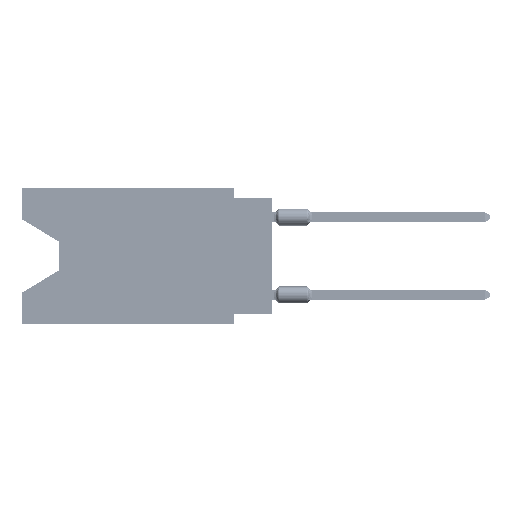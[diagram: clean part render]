
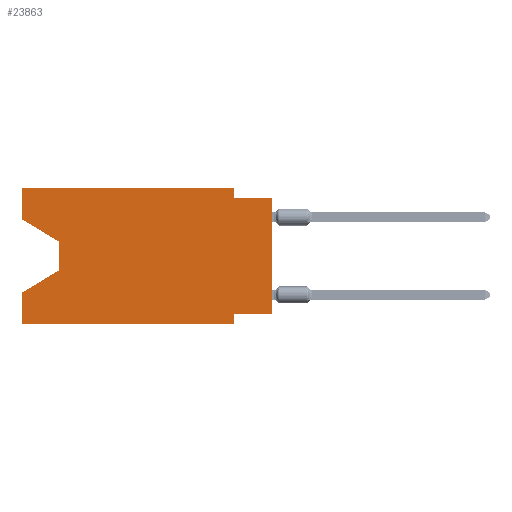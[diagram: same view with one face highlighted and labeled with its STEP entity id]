
A CAD part, left-side view. The second image highlights one B-rep face of the part: STEP entity #23863.
In plain terms, the highlighted planar face has unit normal (-1, 0, 0).
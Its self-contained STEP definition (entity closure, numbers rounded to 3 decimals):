
#1742 = CARTESIAN_POINT ( 'NONE',  ( 0., 2.54, -8.255 ) ) ;
#2446 = VECTOR ( 'NONE', #30770, 1000. ) ;
#2973 = CARTESIAN_POINT ( 'NONE',  ( 0., 16.383, -8.89 ) ) ;
#3612 = LINE ( 'NONE', #27703, #12049 ) ;
#5182 = VECTOR ( 'NONE', #40674, 1000. ) ;
#5457 = VECTOR ( 'NONE', #11142, 1000. ) ;
#6233 = DIRECTION ( 'NONE',  ( 0., 0.855, -0.519 ) ) ;
#7400 = ORIENTED_EDGE ( 'NONE', *, *, #13362, .T. ) ;
#8793 = CARTESIAN_POINT ( 'NONE',  ( 0., 0., -8.255 ) ) ;
#9282 = VECTOR ( 'NONE', #62276, 1000. ) ;
#10349 = CARTESIAN_POINT ( 'NONE',  ( 0., 16.383, 0. ) ) ;
#11142 = DIRECTION ( 'NONE',  ( 0., -1., 0. ) ) ;
#11326 = VERTEX_POINT ( 'NONE', #20243 ) ;
#12049 = VECTOR ( 'NONE', #64136, 1000. ) ;
#12769 = LINE ( 'NONE', #33821, #49837 ) ;
#12831 = EDGE_CURVE ( 'NONE', #11326, #19096, #44899, .T. ) ;
#13362 = EDGE_CURVE ( 'NONE', #62765, #40197, #60546, .T. ) ;
#13784 = VERTEX_POINT ( 'NONE', #51391 ) ;
#14406 = EDGE_CURVE ( 'NONE', #13784, #57135, #62645, .T. ) ;
#14707 = CARTESIAN_POINT ( 'NONE',  ( 0., 13.97, -3.505 ) ) ;
#15293 = VERTEX_POINT ( 'NONE', #64117 ) ;
#15340 = PLANE ( 'NONE',  #50433 ) ;
#15736 = ORIENTED_EDGE ( 'NONE', *, *, #29027, .T. ) ;
#16258 = CARTESIAN_POINT ( 'NONE',  ( 0., 13.97, -3.505 ) ) ;
#17633 = LINE ( 'NONE', #53420, #43109 ) ;
#17650 = DIRECTION ( 'NONE',  ( 0., -1., 0. ) ) ;
#17716 = VERTEX_POINT ( 'NONE', #20116 ) ;
#18101 = DIRECTION ( 'NONE',  ( 0., 0., 1. ) ) ;
#18464 = DIRECTION ( 'NONE',  ( 0., 1., 0. ) ) ;
#19096 = VERTEX_POINT ( 'NONE', #1742 ) ;
#19259 = CARTESIAN_POINT ( 'NONE',  ( 0., 2.54, -8.89 ) ) ;
#20116 = CARTESIAN_POINT ( 'NONE',  ( 0., 2.54, 0. ) ) ;
#20243 = CARTESIAN_POINT ( 'NONE',  ( 0., 0., -8.255 ) ) ;
#20269 = LINE ( 'NONE', #41357, #5182 ) ;
#20420 = CARTESIAN_POINT ( 'NONE',  ( 0., 16.383, 0. ) ) ;
#20440 = ORIENTED_EDGE ( 'NONE', *, *, #31009, .F. ) ;
#20496 = EDGE_CURVE ( 'NONE', #43313, #17716, #59369, .T. ) ;
#20549 = VECTOR ( 'NONE', #6233, 1000. ) ;
#22335 = DIRECTION ( 'NONE',  ( 0., 0., 1. ) ) ;
#23863 = ADVANCED_FACE ( 'NONE', ( #45126 ), #15340, .F. ) ;
#24087 = EDGE_CURVE ( 'NONE', #44730, #15293, #3612, .T. ) ;
#24464 = VERTEX_POINT ( 'NONE', #19259 ) ;
#26157 = LINE ( 'NONE', #46225, #9282 ) ;
#26672 = CARTESIAN_POINT ( 'NONE',  ( 0., 0., -0.635 ) ) ;
#27098 = ORIENTED_EDGE ( 'NONE', *, *, #41077, .F. ) ;
#27703 = CARTESIAN_POINT ( 'NONE',  ( 0., 16.383, 0. ) ) ;
#29027 = EDGE_CURVE ( 'NONE', #11326, #57135, #12769, .T. ) ;
#30283 = CARTESIAN_POINT ( 'NONE',  ( 0., 13.97, -5.385 ) ) ;
#30749 = DIRECTION ( 'NONE',  ( 1., 0., 0. ) ) ;
#30770 = DIRECTION ( 'NONE',  ( 0., 0., -1. ) ) ;
#31009 = EDGE_CURVE ( 'NONE', #56898, #43313, #17633, .T. ) ;
#31687 = ORIENTED_EDGE ( 'NONE', *, *, #12831, .F. ) ;
#33821 = CARTESIAN_POINT ( 'NONE',  ( 0., 0., 0. ) ) ;
#36371 = CARTESIAN_POINT ( 'NONE',  ( 0., 16.383, -2.038 ) ) ;
#38062 = CARTESIAN_POINT ( 'NONE',  ( 0., 16.383, -8.89 ) ) ;
#38403 = LINE ( 'NONE', #2973, #63183 ) ;
#38448 = EDGE_CURVE ( 'NONE', #40197, #15293, #65755, .T. ) ;
#40197 = VERTEX_POINT ( 'NONE', #50184 ) ;
#40674 = DIRECTION ( 'NONE',  ( 0., -0.855, -0.519 ) ) ;
#41077 = EDGE_CURVE ( 'NONE', #17716, #13784, #50035, .T. ) ;
#41095 = VECTOR ( 'NONE', #64768, 1000. ) ;
#41357 = CARTESIAN_POINT ( 'NONE',  ( 0., 16.383, -2.038 ) ) ;
#43109 = VECTOR ( 'NONE', #22335, 1000. ) ;
#43313 = VERTEX_POINT ( 'NONE', #20420 ) ;
#43327 = CARTESIAN_POINT ( 'NONE',  ( 0., 16.383, 0. ) ) ;
#44730 = VERTEX_POINT ( 'NONE', #38062 ) ;
#44813 = DIRECTION ( 'NONE',  ( 0., 0., -1. ) ) ;
#44899 = LINE ( 'NONE', #8793, #61445 ) ;
#44969 = ORIENTED_EDGE ( 'NONE', *, *, #38448, .T. ) ;
#45126 = FACE_OUTER_BOUND ( 'NONE', #49831, .T. ) ;
#45675 = CARTESIAN_POINT ( 'NONE',  ( 0., 2.54, 0. ) ) ;
#46225 = CARTESIAN_POINT ( 'NONE',  ( 0., 2.54, -8.89 ) ) ;
#46554 = EDGE_CURVE ( 'NONE', #44730, #24464, #38403, .T. ) ;
#46617 = ORIENTED_EDGE ( 'NONE', *, *, #20496, .F. ) ;
#46936 = CARTESIAN_POINT ( 'NONE',  ( 0., 0., -0.635 ) ) ;
#49831 = EDGE_LOOP ( 'NONE', ( #62853, #7400, #44969, #55648, #59525, #50130, #31687, #15736, #64018, #27098, #46617, #20440 ) ) ;
#49837 = VECTOR ( 'NONE', #18101, 1000. ) ;
#50035 = LINE ( 'NONE', #45675, #41095 ) ;
#50130 = ORIENTED_EDGE ( 'NONE', *, *, #56031, .F. ) ;
#50184 = CARTESIAN_POINT ( 'NONE',  ( 0., 13.97, -5.385 ) ) ;
#50433 = AXIS2_PLACEMENT_3D ( 'NONE', #10349, #30749, #44813 ) ;
#51391 = CARTESIAN_POINT ( 'NONE',  ( 0., 2.54, -0.635 ) ) ;
#53420 = CARTESIAN_POINT ( 'NONE',  ( 0., 16.383, 0. ) ) ;
#55648 = ORIENTED_EDGE ( 'NONE', *, *, #24087, .F. ) ;
#56031 = EDGE_CURVE ( 'NONE', #19096, #24464, #26157, .T. ) ;
#56075 = VECTOR ( 'NONE', #63738, 1000. ) ;
#56898 = VERTEX_POINT ( 'NONE', #36371 ) ;
#57135 = VERTEX_POINT ( 'NONE', #26672 ) ;
#59369 = LINE ( 'NONE', #43327, #56075 ) ;
#59525 = ORIENTED_EDGE ( 'NONE', *, *, #46554, .T. ) ;
#60546 = LINE ( 'NONE', #14707, #2446 ) ;
#61445 = VECTOR ( 'NONE', #18464, 1000. ) ;
#61560 = EDGE_CURVE ( 'NONE', #56898, #62765, #20269, .T. ) ;
#62276 = DIRECTION ( 'NONE',  ( 0., 0., -1. ) ) ;
#62645 = LINE ( 'NONE', #46936, #5457 ) ;
#62765 = VERTEX_POINT ( 'NONE', #16258 ) ;
#62853 = ORIENTED_EDGE ( 'NONE', *, *, #61560, .T. ) ;
#63183 = VECTOR ( 'NONE', #17650, 1000. ) ;
#63738 = DIRECTION ( 'NONE',  ( 0., -1., 0. ) ) ;
#64018 = ORIENTED_EDGE ( 'NONE', *, *, #14406, .F. ) ;
#64117 = CARTESIAN_POINT ( 'NONE',  ( 0., 16.383, -6.852 ) ) ;
#64136 = DIRECTION ( 'NONE',  ( 0., 0., 1. ) ) ;
#64768 = DIRECTION ( 'NONE',  ( 0., 0., -1. ) ) ;
#65755 = LINE ( 'NONE', #30283, #20549 ) ;
